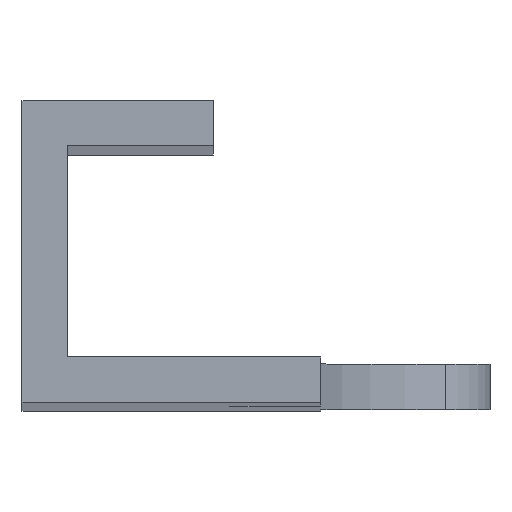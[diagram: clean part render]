
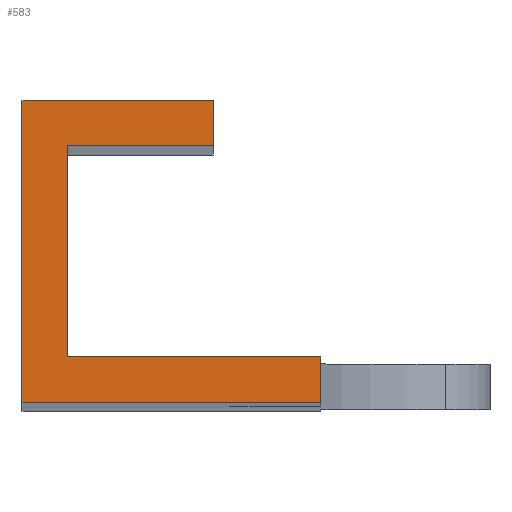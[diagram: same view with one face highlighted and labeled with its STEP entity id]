
A CAD part, top view. The second image highlights one B-rep face of the part: STEP entity #583.
In plain terms, the highlighted planar face has unit normal (0, 0, 1).
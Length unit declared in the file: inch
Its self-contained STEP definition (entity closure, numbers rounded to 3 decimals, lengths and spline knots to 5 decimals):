
#39=PLANE('',#634);
#58=FACE_OUTER_BOUND('',#85,.T.);
#85=EDGE_LOOP('',(#455,#456,#457,#458,#459,#460,#461,#462));
#125=LINE('',#864,#180);
#140=LINE('',#898,#195);
#148=LINE('',#913,#203);
#149=LINE('',#916,#204);
#150=LINE('',#918,#205);
#151=LINE('',#920,#206);
#152=LINE('',#922,#207);
#153=LINE('',#923,#208);
#180=VECTOR('',#692,0.3937);
#195=VECTOR('',#719,0.3937);
#203=VECTOR('',#735,0.3937);
#204=VECTOR('',#738,0.3937);
#205=VECTOR('',#739,0.3937);
#206=VECTOR('',#740,0.3937);
#207=VECTOR('',#741,0.3937);
#208=VECTOR('',#742,0.3937);
#264=VERTEX_POINT('',#861);
#265=VERTEX_POINT('',#863);
#277=VERTEX_POINT('',#895);
#278=VERTEX_POINT('',#897);
#282=VERTEX_POINT('',#915);
#283=VERTEX_POINT('',#917);
#284=VERTEX_POINT('',#919);
#285=VERTEX_POINT('',#921);
#323=EDGE_CURVE('',#264,#265,#125,.T.);
#340=EDGE_CURVE('',#277,#278,#140,.T.);
#348=EDGE_CURVE('',#265,#277,#148,.T.);
#349=EDGE_CURVE('',#282,#264,#149,.T.);
#350=EDGE_CURVE('',#283,#282,#150,.T.);
#351=EDGE_CURVE('',#284,#283,#151,.T.);
#352=EDGE_CURVE('',#285,#284,#152,.T.);
#353=EDGE_CURVE('',#278,#285,#153,.T.);
#455=ORIENTED_EDGE('',*,*,#348,.F.);
#456=ORIENTED_EDGE('',*,*,#323,.F.);
#457=ORIENTED_EDGE('',*,*,#349,.F.);
#458=ORIENTED_EDGE('',*,*,#350,.F.);
#459=ORIENTED_EDGE('',*,*,#351,.F.);
#460=ORIENTED_EDGE('',*,*,#352,.F.);
#461=ORIENTED_EDGE('',*,*,#353,.F.);
#462=ORIENTED_EDGE('',*,*,#340,.F.);
#583=ADVANCED_FACE('',(#58),#39,.F.);
#634=AXIS2_PLACEMENT_3D('',#914,#736,#737);
#692=DIRECTION('',(1.,0.,0.));
#719=DIRECTION('',(-1.,0.,0.));
#735=DIRECTION('',(0.,-1.,0.));
#736=DIRECTION('center_axis',(0.,0.,-1.));
#737=DIRECTION('ref_axis',(-1.,0.,0.));
#738=DIRECTION('',(0.,-1.,0.));
#739=DIRECTION('',(-1.,0.,0.));
#740=DIRECTION('',(0.,-1.,0.));
#741=DIRECTION('',(1.,0.,0.));
#742=DIRECTION('',(0.,1.,0.));
#861=CARTESIAN_POINT('',(-0.33094,0.05906,6.80194));
#863=CARTESIAN_POINT('',(0.,0.05906,6.80194));
#864=CARTESIAN_POINT('',(-0.0975,0.05906,6.80194));
#895=CARTESIAN_POINT('',(0.,0.,6.80194));
#897=CARTESIAN_POINT('',(-0.39,0.,6.80194));
#898=CARTESIAN_POINT('',(-0.2925,0.,6.80194));
#913=CARTESIAN_POINT('',(0.,0.09843,6.80194));
#914=CARTESIAN_POINT('Origin',(-0.195,0.19685,6.80194));
#915=CARTESIAN_POINT('',(-0.33094,0.33465,6.80194));
#916=CARTESIAN_POINT('',(-0.33094,0.12795,6.80194));
#917=CARTESIAN_POINT('',(-0.14,0.33465,6.80194));
#918=CARTESIAN_POINT('',(-0.26297,0.33465,6.80194));
#919=CARTESIAN_POINT('',(-0.14,0.3937,6.80194));
#920=CARTESIAN_POINT('',(-0.14,0.29528,6.80194));
#921=CARTESIAN_POINT('',(-0.39,0.3937,6.80194));
#922=CARTESIAN_POINT('',(-0.1525,0.3937,6.80194));
#923=CARTESIAN_POINT('',(-0.39,0.29528,6.80194));
